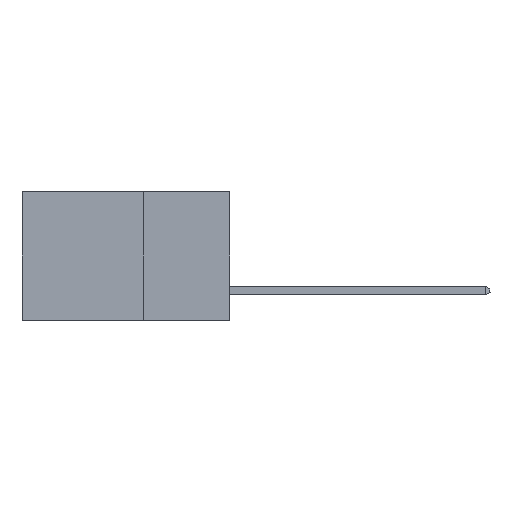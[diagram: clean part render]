
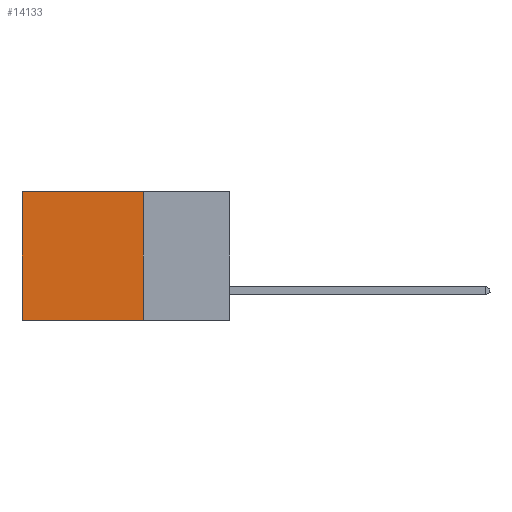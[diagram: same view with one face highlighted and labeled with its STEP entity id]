
A CAD part, left-side view. The second image highlights one B-rep face of the part: STEP entity #14133.
In plain terms, the highlighted planar face has unit normal (-1, 0, 0).
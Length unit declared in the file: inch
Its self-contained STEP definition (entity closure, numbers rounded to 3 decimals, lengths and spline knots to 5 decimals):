
#1245 = VECTOR ( 'NONE', #4616, 39.37008 ) ;
#1746 = LINE ( 'NONE', #11497, #3861 ) ;
#3331 = EDGE_CURVE ( 'NONE', #12266, #11067, #19996, .T. ) ;
#3824 = VERTEX_POINT ( 'NONE', #10260 ) ;
#3861 = VECTOR ( 'NONE', #13275, 39.37008 ) ;
#4616 = DIRECTION ( 'NONE',  ( 0., 0., -1. ) ) ;
#5137 = DIRECTION ( 'NONE',  ( 0., 1., 0. ) ) ;
#6844 = VECTOR ( 'NONE', #5137, 39.37008 ) ;
#8580 = CARTESIAN_POINT ( 'NONE',  ( 0.298, 0.25, 0. ) ) ;
#8780 = AXIS2_PLACEMENT_3D ( 'NONE', #8580, #22012, #12358 ) ;
#9496 = CARTESIAN_POINT ( 'NONE',  ( 0.298, 0.25, -0.37 ) ) ;
#9655 = CARTESIAN_POINT ( 'NONE',  ( 0.298, 0.6, -0.37 ) ) ;
#10260 = CARTESIAN_POINT ( 'NONE',  ( 0.298, 0.25, 0. ) ) ;
#11067 = VERTEX_POINT ( 'NONE', #9655 ) ;
#11317 = ORIENTED_EDGE ( 'NONE', *, *, #3331, .T. ) ;
#11497 = CARTESIAN_POINT ( 'NONE',  ( 0.298, 0.25, 0. ) ) ;
#12266 = VERTEX_POINT ( 'NONE', #18834 ) ;
#12358 = DIRECTION ( 'NONE',  ( 0., 0., -1. ) ) ;
#12946 = VERTEX_POINT ( 'NONE', #9496 ) ;
#13275 = DIRECTION ( 'NONE',  ( 0., 0., -1. ) ) ;
#14133 = ADVANCED_FACE ( 'NONE', ( #18790 ), #18160, .F. ) ;
#14372 = VECTOR ( 'NONE', #17028, 39.37008 ) ;
#16958 = EDGE_CURVE ( 'NONE', #3824, #12946, #1746, .T. ) ;
#17028 = DIRECTION ( 'NONE',  ( 0., 1., 0. ) ) ;
#17122 = LINE ( 'NONE', #24492, #6844 ) ;
#18160 = PLANE ( 'NONE',  #8780 ) ;
#18315 = ORIENTED_EDGE ( 'NONE', *, *, #22869, .T. ) ;
#18790 = FACE_OUTER_BOUND ( 'NONE', #24578, .T. ) ;
#18834 = CARTESIAN_POINT ( 'NONE',  ( 0.298, 0.6, 0. ) ) ;
#19570 = LINE ( 'NONE', #21007, #14372 ) ;
#19996 = LINE ( 'NONE', #20088, #1245 ) ;
#20088 = CARTESIAN_POINT ( 'NONE',  ( 0.298, 0.6, 0. ) ) ;
#20549 = ORIENTED_EDGE ( 'NONE', *, *, #22279, .F. ) ;
#21007 = CARTESIAN_POINT ( 'NONE',  ( 0.298, 0.25, -0.37 ) ) ;
#22012 = DIRECTION ( 'NONE',  ( 1., 0., 0. ) ) ;
#22279 = EDGE_CURVE ( 'NONE', #12946, #11067, #19570, .T. ) ;
#22869 = EDGE_CURVE ( 'NONE', #3824, #12266, #17122, .T. ) ;
#23941 = ORIENTED_EDGE ( 'NONE', *, *, #16958, .F. ) ;
#24492 = CARTESIAN_POINT ( 'NONE',  ( 0.298, 0.25, 0. ) ) ;
#24578 = EDGE_LOOP ( 'NONE', ( #11317, #20549, #23941, #18315 ) ) ;
